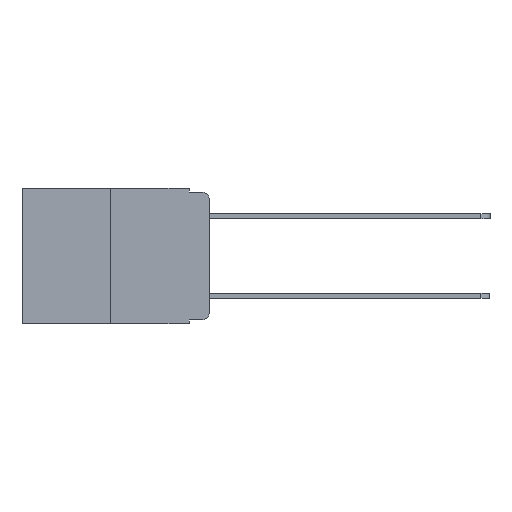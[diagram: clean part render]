
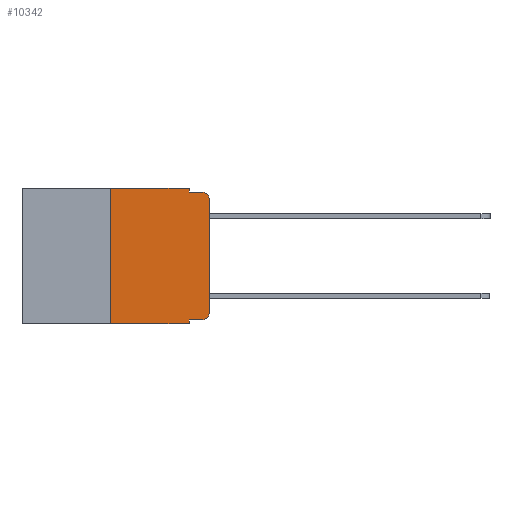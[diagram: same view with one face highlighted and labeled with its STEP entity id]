
A CAD part, left-side view. The second image highlights one B-rep face of the part: STEP entity #10342.
In plain terms, the highlighted planar face has unit normal (-1, 0, 0).
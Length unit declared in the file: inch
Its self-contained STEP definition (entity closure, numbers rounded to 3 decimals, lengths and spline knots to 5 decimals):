
#340 = CARTESIAN_POINT ( 'NONE',  ( 0., 0.25, 0. ) ) ;
#538 = CARTESIAN_POINT ( 'NONE',  ( 0., 0.02, -0.313 ) ) ;
#548 = FACE_OUTER_BOUND ( 'NONE', #10763, .T. ) ;
#927 = VERTEX_POINT ( 'NONE', #5683 ) ;
#936 = AXIS2_PLACEMENT_3D ( 'NONE', #2975, #17332, #5111 ) ;
#2616 = VECTOR ( 'NONE', #16615, 39.37008 ) ;
#2692 = DIRECTION ( 'NONE',  ( 0., 0., -1. ) ) ;
#2848 = CARTESIAN_POINT ( 'NONE',  ( 0., 0.25, 0. ) ) ;
#2975 = CARTESIAN_POINT ( 'NONE',  ( 0., 0.02, -0.03 ) ) ;
#3701 = VERTEX_POINT ( 'NONE', #21186 ) ;
#3789 = EDGE_CURVE ( 'NONE', #17323, #6362, #4863, .T. ) ;
#4202 = VECTOR ( 'NONE', #6417, 39.37008 ) ;
#4863 = CIRCLE ( 'NONE', #936, 0.02 ) ;
#5111 = DIRECTION ( 'NONE',  ( 0., 0., -1. ) ) ;
#5325 = ORIENTED_EDGE ( 'NONE', *, *, #13042, .F. ) ;
#5367 = LINE ( 'NONE', #16818, #21670 ) ;
#5683 = CARTESIAN_POINT ( 'NONE',  ( 0., 0.25, -0.343 ) ) ;
#5721 = EDGE_CURVE ( 'NONE', #3701, #15000, #10891, .T. ) ;
#6253 = CARTESIAN_POINT ( 'NONE',  ( 0., 0.051, -0.01 ) ) ;
#6362 = VERTEX_POINT ( 'NONE', #15003 ) ;
#6417 = DIRECTION ( 'NONE',  ( 0., 0., -1. ) ) ;
#6978 = DIRECTION ( 'NONE',  ( 0., -1., 0. ) ) ;
#7389 = CARTESIAN_POINT ( 'NONE',  ( 0., 0.473, -0.343 ) ) ;
#9129 = CARTESIAN_POINT ( 'NONE',  ( 0., 0.051, -0.01 ) ) ;
#9334 = EDGE_CURVE ( 'NONE', #20371, #17323, #13640, .T. ) ;
#9521 = DIRECTION ( 'NONE',  ( 0., 0., -1. ) ) ;
#9538 = CIRCLE ( 'NONE', #22810, 0.02 ) ;
#10211 = CARTESIAN_POINT ( 'NONE',  ( 0., 0., -0.03 ) ) ;
#10342 = ADVANCED_FACE ( 'NONE', ( #548 ), #20164, .F. ) ;
#10763 = EDGE_LOOP ( 'NONE', ( #22427, #11973, #18957, #11713, #5325, #13935, #18703, #15277, #15616, #13400 ) ) ;
#10809 = CARTESIAN_POINT ( 'NONE',  ( 0., 0.051, -0.333 ) ) ;
#10891 = LINE ( 'NONE', #17291, #16302 ) ;
#11713 = ORIENTED_EDGE ( 'NONE', *, *, #22138, .F. ) ;
#11973 = ORIENTED_EDGE ( 'NONE', *, *, #3789, .T. ) ;
#12003 = CARTESIAN_POINT ( 'NONE',  ( 0., 0.473, 0. ) ) ;
#12091 = DIRECTION ( 'NONE',  ( 1., 0., 0. ) ) ;
#12570 = CARTESIAN_POINT ( 'NONE',  ( 0., 0., 0. ) ) ;
#13042 = EDGE_CURVE ( 'NONE', #20173, #18834, #5367, .T. ) ;
#13120 = EDGE_CURVE ( 'NONE', #17829, #20371, #9538, .T. ) ;
#13400 = ORIENTED_EDGE ( 'NONE', *, *, #13120, .T. ) ;
#13572 = DIRECTION ( 'NONE',  ( 0., -1., 0. ) ) ;
#13640 = LINE ( 'NONE', #12570, #2616 ) ;
#13857 = CARTESIAN_POINT ( 'NONE',  ( 0., 0., -0.313 ) ) ;
#13935 = ORIENTED_EDGE ( 'NONE', *, *, #19418, .F. ) ;
#14408 = LINE ( 'NONE', #9129, #19832 ) ;
#14754 = VECTOR ( 'NONE', #14878, 39.37008 ) ;
#14878 = DIRECTION ( 'NONE',  ( 0., 0., 1. ) ) ;
#15000 = VERTEX_POINT ( 'NONE', #18999 ) ;
#15003 = CARTESIAN_POINT ( 'NONE',  ( 0., 0.02, -0.01 ) ) ;
#15069 = DIRECTION ( 'NONE',  ( -1., 0., 0. ) ) ;
#15277 = ORIENTED_EDGE ( 'NONE', *, *, #5721, .F. ) ;
#15386 = LINE ( 'NONE', #10809, #18852 ) ;
#15616 = ORIENTED_EDGE ( 'NONE', *, *, #23986, .T. ) ;
#15865 = EDGE_CURVE ( 'NONE', #927, #15000, #21954, .T. ) ;
#16302 = VECTOR ( 'NONE', #19360, 39.37008 ) ;
#16615 = DIRECTION ( 'NONE',  ( 0., 0., 1. ) ) ;
#16818 = CARTESIAN_POINT ( 'NONE',  ( 0., 0.473, 0. ) ) ;
#17291 = CARTESIAN_POINT ( 'NONE',  ( 0., 0.051, 0. ) ) ;
#17323 = VERTEX_POINT ( 'NONE', #10211 ) ;
#17332 = DIRECTION ( 'NONE',  ( -1., 0., 0. ) ) ;
#17423 = CARTESIAN_POINT ( 'NONE',  ( 0., 0.02, -0.333 ) ) ;
#17472 = VECTOR ( 'NONE', #13572, 39.37008 ) ;
#17829 = VERTEX_POINT ( 'NONE', #17423 ) ;
#18623 = CARTESIAN_POINT ( 'NONE',  ( 0., 0.051, 0. ) ) ;
#18703 = ORIENTED_EDGE ( 'NONE', *, *, #15865, .T. ) ;
#18834 = VERTEX_POINT ( 'NONE', #22466 ) ;
#18852 = VECTOR ( 'NONE', #25001, 39.37008 ) ;
#18957 = ORIENTED_EDGE ( 'NONE', *, *, #23499, .F. ) ;
#18999 = CARTESIAN_POINT ( 'NONE',  ( 0., 0.051, -0.343 ) ) ;
#19360 = DIRECTION ( 'NONE',  ( 0., 0., -1. ) ) ;
#19418 = EDGE_CURVE ( 'NONE', #927, #20173, #26141, .T. ) ;
#19832 = VECTOR ( 'NONE', #6978, 39.37008 ) ;
#20164 = PLANE ( 'NONE',  #23278 ) ;
#20173 = VERTEX_POINT ( 'NONE', #2848 ) ;
#20371 = VERTEX_POINT ( 'NONE', #13857 ) ;
#20940 = DIRECTION ( 'NONE',  ( 0., -1., 0. ) ) ;
#21182 = LINE ( 'NONE', #18623, #4202 ) ;
#21186 = CARTESIAN_POINT ( 'NONE',  ( 0., 0.051, -0.333 ) ) ;
#21670 = VECTOR ( 'NONE', #20940, 39.37008 ) ;
#21954 = LINE ( 'NONE', #7389, #17472 ) ;
#22138 = EDGE_CURVE ( 'NONE', #18834, #25933, #21182, .T. ) ;
#22427 = ORIENTED_EDGE ( 'NONE', *, *, #9334, .T. ) ;
#22466 = CARTESIAN_POINT ( 'NONE',  ( 0., 0.051, 0. ) ) ;
#22810 = AXIS2_PLACEMENT_3D ( 'NONE', #538, #15069, #2692 ) ;
#23278 = AXIS2_PLACEMENT_3D ( 'NONE', #12003, #12091, #9521 ) ;
#23499 = EDGE_CURVE ( 'NONE', #25933, #6362, #14408, .T. ) ;
#23986 = EDGE_CURVE ( 'NONE', #3701, #17829, #15386, .T. ) ;
#25001 = DIRECTION ( 'NONE',  ( 0., -1., 0. ) ) ;
#25933 = VERTEX_POINT ( 'NONE', #6253 ) ;
#26141 = LINE ( 'NONE', #340, #14754 ) ;
